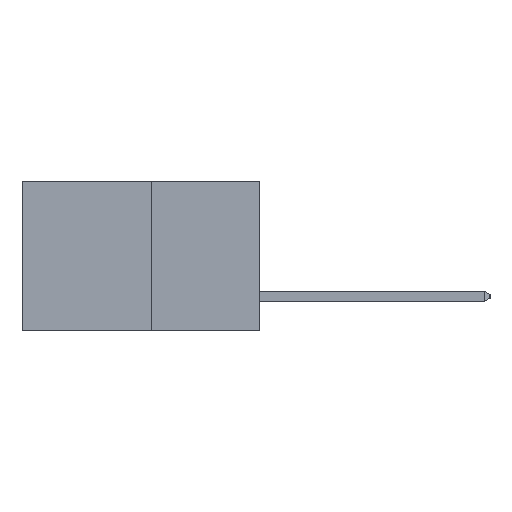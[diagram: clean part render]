
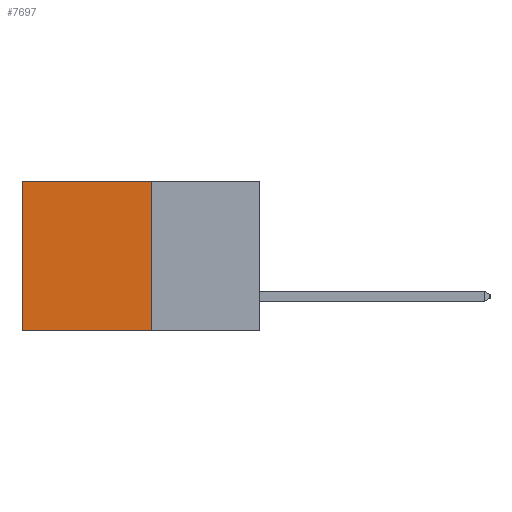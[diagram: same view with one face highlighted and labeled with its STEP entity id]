
A CAD part, left-side view. The second image highlights one B-rep face of the part: STEP entity #7697.
In plain terms, the highlighted planar face has unit normal (-1, 0, 0).
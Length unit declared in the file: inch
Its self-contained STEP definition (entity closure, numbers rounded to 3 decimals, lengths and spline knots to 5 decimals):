
#398 = CARTESIAN_POINT ( 'NONE',  ( 0.277, 0.27, -0.37 ) ) ;
#440 = DIRECTION ( 'NONE',  ( 1., 0., 0. ) ) ;
#725 = VERTEX_POINT ( 'NONE', #6512 ) ;
#821 = CARTESIAN_POINT ( 'NONE',  ( 0.277, 0.27, -0.37 ) ) ;
#1263 = VERTEX_POINT ( 'NONE', #9361 ) ;
#1431 = AXIS2_PLACEMENT_3D ( 'NONE', #398, #440, #7467 ) ;
#1869 = DIRECTION ( 'NONE',  ( 0., 1., 0. ) ) ;
#1914 = DIRECTION ( 'NONE',  ( 0., 0., -1. ) ) ;
#2700 = DIRECTION ( 'NONE',  ( 0., 1., 0. ) ) ;
#3619 = LINE ( 'NONE', #821, #11153 ) ;
#3818 = VERTEX_POINT ( 'NONE', #11016 ) ;
#4711 = FACE_OUTER_BOUND ( 'NONE', #5654, .T. ) ;
#5062 = VECTOR ( 'NONE', #7626, 39.37008 ) ;
#5240 = LINE ( 'NONE', #12490, #10132 ) ;
#5337 = ORIENTED_EDGE ( 'NONE', *, *, #5980, .T. ) ;
#5654 = EDGE_LOOP ( 'NONE', ( #5337, #8182, #6025, #11026 ) ) ;
#5815 = EDGE_CURVE ( 'NONE', #725, #3818, #5240, .T. ) ;
#5980 = EDGE_CURVE ( 'NONE', #3818, #1263, #8332, .T. ) ;
#6023 = VECTOR ( 'NONE', #1914, 39.37008 ) ;
#6025 = ORIENTED_EDGE ( 'NONE', *, *, #10056, .F. ) ;
#6243 = CARTESIAN_POINT ( 'NONE',  ( 0.277, 0.27, -0.37 ) ) ;
#6512 = CARTESIAN_POINT ( 'NONE',  ( 0.277, 0.27, 0. ) ) ;
#7467 = DIRECTION ( 'NONE',  ( 0., 0., -1. ) ) ;
#7626 = DIRECTION ( 'NONE',  ( 0., 0., -1. ) ) ;
#7697 = ADVANCED_FACE ( 'NONE', ( #4711 ), #12243, .F. ) ;
#7712 = LINE ( 'NONE', #9502, #5062 ) ;
#8182 = ORIENTED_EDGE ( 'NONE', *, *, #10424, .F. ) ;
#8332 = LINE ( 'NONE', #11750, #6023 ) ;
#9361 = CARTESIAN_POINT ( 'NONE',  ( 0.277, 0.59, -0.37 ) ) ;
#9502 = CARTESIAN_POINT ( 'NONE',  ( 0.277, 0.27, -0.37 ) ) ;
#10056 = EDGE_CURVE ( 'NONE', #725, #12579, #7712, .T. ) ;
#10132 = VECTOR ( 'NONE', #2700, 39.37008 ) ;
#10424 = EDGE_CURVE ( 'NONE', #12579, #1263, #3619, .T. ) ;
#11016 = CARTESIAN_POINT ( 'NONE',  ( 0.277, 0.59, 0. ) ) ;
#11026 = ORIENTED_EDGE ( 'NONE', *, *, #5815, .T. ) ;
#11153 = VECTOR ( 'NONE', #1869, 39.37008 ) ;
#11750 = CARTESIAN_POINT ( 'NONE',  ( 0.277, 0.59, -0.37 ) ) ;
#12243 = PLANE ( 'NONE',  #1431 ) ;
#12490 = CARTESIAN_POINT ( 'NONE',  ( 0.277, 0.27, 0. ) ) ;
#12579 = VERTEX_POINT ( 'NONE', #6243 ) ;
